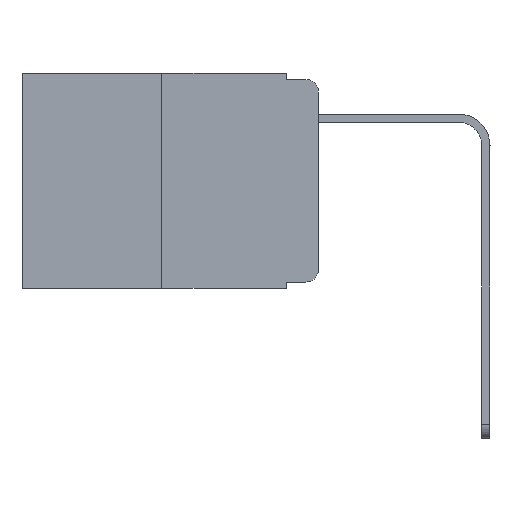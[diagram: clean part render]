
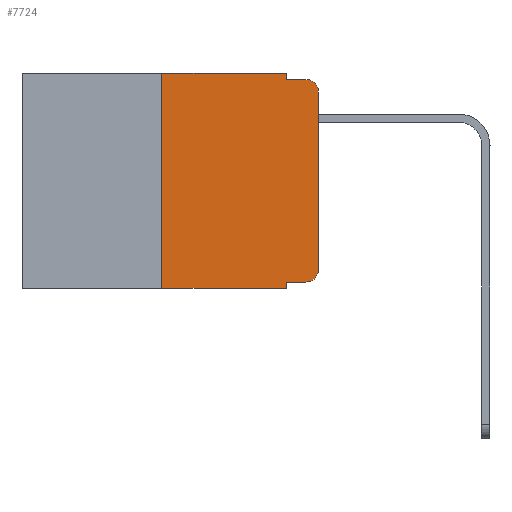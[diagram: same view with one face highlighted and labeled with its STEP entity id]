
A CAD part, left-side view. The second image highlights one B-rep face of the part: STEP entity #7724.
In plain terms, the highlighted planar face has unit normal (-1, 0, 0).
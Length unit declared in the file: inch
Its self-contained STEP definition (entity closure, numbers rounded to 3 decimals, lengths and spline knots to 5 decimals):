
#279 = DIRECTION ( 'NONE',  ( 0., -1., 0. ) ) ;
#851 = CARTESIAN_POINT ( 'NONE',  ( 0., 0., -0.313 ) ) ;
#980 = CARTESIAN_POINT ( 'NONE',  ( 0., 0.473, 0. ) ) ;
#1034 = CARTESIAN_POINT ( 'NONE',  ( 0., 0.473, -0.343 ) ) ;
#1140 = LINE ( 'NONE', #12914, #5963 ) ;
#1743 = VECTOR ( 'NONE', #7602, 39.37008 ) ;
#1760 = VECTOR ( 'NONE', #4344, 39.37008 ) ;
#1772 = DIRECTION ( 'NONE',  ( 0., 0., -1. ) ) ;
#1871 = VECTOR ( 'NONE', #17823, 39.37008 ) ;
#1909 = ORIENTED_EDGE ( 'NONE', *, *, #7155, .F. ) ;
#1922 = CIRCLE ( 'NONE', #4736, 0.02 ) ;
#2169 = AXIS2_PLACEMENT_3D ( 'NONE', #10909, #11109, #9604 ) ;
#2778 = ORIENTED_EDGE ( 'NONE', *, *, #9127, .F. ) ;
#3001 = CARTESIAN_POINT ( 'NONE',  ( 0., 0.051, -0.333 ) ) ;
#3229 = LINE ( 'NONE', #1034, #4975 ) ;
#4157 = VECTOR ( 'NONE', #279, 39.37008 ) ;
#4344 = DIRECTION ( 'NONE',  ( 0., -1., 0. ) ) ;
#4404 = DIRECTION ( 'NONE',  ( 0., 0., 1. ) ) ;
#4594 = EDGE_CURVE ( 'NONE', #13995, #14708, #1922, .T. ) ;
#4736 = AXIS2_PLACEMENT_3D ( 'NONE', #9483, #6765, #16448 ) ;
#4786 = CARTESIAN_POINT ( 'NONE',  ( 0., 0.051, -0.343 ) ) ;
#4975 = VECTOR ( 'NONE', #17812, 39.37008 ) ;
#5032 = LINE ( 'NONE', #15672, #4157 ) ;
#5086 = CARTESIAN_POINT ( 'NONE',  ( 0., 0.02, -0.333 ) ) ;
#5104 = LINE ( 'NONE', #17889, #14560 ) ;
#5510 = ORIENTED_EDGE ( 'NONE', *, *, #14955, .T. ) ;
#5521 = ORIENTED_EDGE ( 'NONE', *, *, #6061, .F. ) ;
#5619 = EDGE_CURVE ( 'NONE', #14708, #15384, #6683, .T. ) ;
#5963 = VECTOR ( 'NONE', #4404, 39.37008 ) ;
#6061 = EDGE_CURVE ( 'NONE', #15057, #15371, #13945, .T. ) ;
#6229 = ORIENTED_EDGE ( 'NONE', *, *, #10700, .F. ) ;
#6294 = ORIENTED_EDGE ( 'NONE', *, *, #16090, .F. ) ;
#6651 = VERTEX_POINT ( 'NONE', #16932 ) ;
#6683 = LINE ( 'NONE', #14858, #1871 ) ;
#6765 = DIRECTION ( 'NONE',  ( -1., 0., 0. ) ) ;
#6803 = DIRECTION ( 'NONE',  ( 0., 0., -1. ) ) ;
#7155 = EDGE_CURVE ( 'NONE', #10082, #14774, #5104, .T. ) ;
#7602 = DIRECTION ( 'NONE',  ( 0., -1., 0. ) ) ;
#7724 = ADVANCED_FACE ( 'NONE', ( #17188 ), #12101, .F. ) ;
#8025 = CARTESIAN_POINT ( 'NONE',  ( 0., 0.051, -0.01 ) ) ;
#8034 = DIRECTION ( 'NONE',  ( 0., 0., -1. ) ) ;
#8444 = VERTEX_POINT ( 'NONE', #15183 ) ;
#8557 = LINE ( 'NONE', #16291, #1743 ) ;
#8992 = CARTESIAN_POINT ( 'NONE',  ( 0., 0.051, 0. ) ) ;
#9127 = EDGE_CURVE ( 'NONE', #14956, #8444, #1140, .T. ) ;
#9438 = ORIENTED_EDGE ( 'NONE', *, *, #10598, .T. ) ;
#9483 = CARTESIAN_POINT ( 'NONE',  ( 0., 0.02, -0.313 ) ) ;
#9547 = CARTESIAN_POINT ( 'NONE',  ( 0., 0.25, -0.343 ) ) ;
#9604 = DIRECTION ( 'NONE',  ( 0., 0., -1. ) ) ;
#10082 = VERTEX_POINT ( 'NONE', #8992 ) ;
#10349 = CARTESIAN_POINT ( 'NONE',  ( 0., 0., -0.03 ) ) ;
#10598 = EDGE_CURVE ( 'NONE', #15057, #13995, #14929, .T. ) ;
#10700 = EDGE_CURVE ( 'NONE', #8444, #10082, #5032, .T. ) ;
#10909 = CARTESIAN_POINT ( 'NONE',  ( 0., 0.02, -0.03 ) ) ;
#11109 = DIRECTION ( 'NONE',  ( -1., 0., 0. ) ) ;
#11738 = CARTESIAN_POINT ( 'NONE',  ( 0., 0.051, 0. ) ) ;
#11936 = EDGE_CURVE ( 'NONE', #14956, #15371, #3229, .T. ) ;
#12101 = PLANE ( 'NONE',  #13846 ) ;
#12914 = CARTESIAN_POINT ( 'NONE',  ( 0., 0.25, 0. ) ) ;
#13123 = ORIENTED_EDGE ( 'NONE', *, *, #11936, .T. ) ;
#13414 = CIRCLE ( 'NONE', #2169, 0.02 ) ;
#13845 = CARTESIAN_POINT ( 'NONE',  ( 0., 0.051, -0.333 ) ) ;
#13846 = AXIS2_PLACEMENT_3D ( 'NONE', #980, #16347, #8034 ) ;
#13945 = LINE ( 'NONE', #11738, #15728 ) ;
#13995 = VERTEX_POINT ( 'NONE', #5086 ) ;
#14560 = VECTOR ( 'NONE', #6803, 39.37008 ) ;
#14708 = VERTEX_POINT ( 'NONE', #851 ) ;
#14774 = VERTEX_POINT ( 'NONE', #8025 ) ;
#14858 = CARTESIAN_POINT ( 'NONE',  ( 0., 0., 0. ) ) ;
#14929 = LINE ( 'NONE', #3001, #1760 ) ;
#14955 = EDGE_CURVE ( 'NONE', #15384, #6651, #13414, .T. ) ;
#14956 = VERTEX_POINT ( 'NONE', #9547 ) ;
#15057 = VERTEX_POINT ( 'NONE', #13845 ) ;
#15183 = CARTESIAN_POINT ( 'NONE',  ( 0., 0.25, 0. ) ) ;
#15371 = VERTEX_POINT ( 'NONE', #4786 ) ;
#15384 = VERTEX_POINT ( 'NONE', #10349 ) ;
#15672 = CARTESIAN_POINT ( 'NONE',  ( 0., 0.473, 0. ) ) ;
#15728 = VECTOR ( 'NONE', #1772, 39.37008 ) ;
#16090 = EDGE_CURVE ( 'NONE', #14774, #6651, #8557, .T. ) ;
#16291 = CARTESIAN_POINT ( 'NONE',  ( 0., 0.051, -0.01 ) ) ;
#16347 = DIRECTION ( 'NONE',  ( 1., 0., 0. ) ) ;
#16448 = DIRECTION ( 'NONE',  ( 0., 0., -1. ) ) ;
#16932 = CARTESIAN_POINT ( 'NONE',  ( 0., 0.02, -0.01 ) ) ;
#17118 = EDGE_LOOP ( 'NONE', ( #18083, #5510, #6294, #1909, #6229, #2778, #13123, #5521, #9438, #17578 ) ) ;
#17188 = FACE_OUTER_BOUND ( 'NONE', #17118, .T. ) ;
#17578 = ORIENTED_EDGE ( 'NONE', *, *, #4594, .T. ) ;
#17812 = DIRECTION ( 'NONE',  ( 0., -1., 0. ) ) ;
#17823 = DIRECTION ( 'NONE',  ( 0., 0., 1. ) ) ;
#17889 = CARTESIAN_POINT ( 'NONE',  ( 0., 0.051, 0. ) ) ;
#18083 = ORIENTED_EDGE ( 'NONE', *, *, #5619, .T. ) ;
